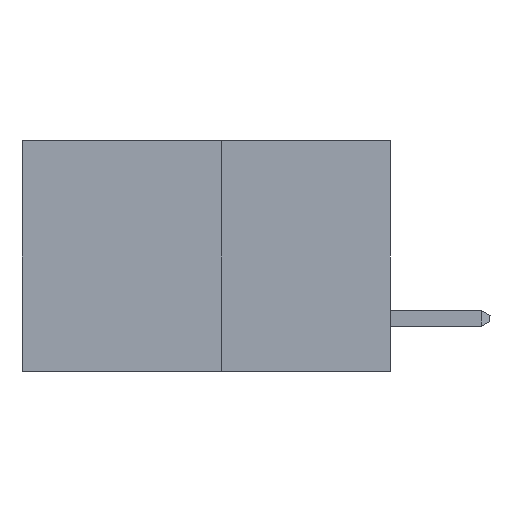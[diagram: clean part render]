
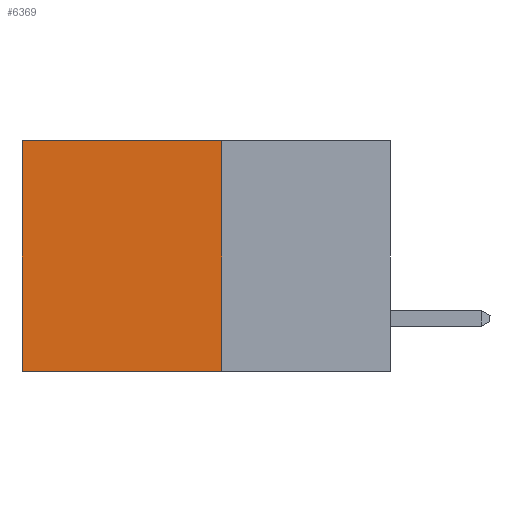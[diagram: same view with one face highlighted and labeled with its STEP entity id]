
A CAD part, left-side view. The second image highlights one B-rep face of the part: STEP entity #6369.
In plain terms, the highlighted planar face has unit normal (-1, 0, 0).
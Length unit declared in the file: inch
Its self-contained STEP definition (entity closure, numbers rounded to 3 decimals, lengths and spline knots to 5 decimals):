
#111 = LINE ( 'NONE', #5739, #2231 ) ;
#535 = VECTOR ( 'NONE', #11121, 39.37008 ) ;
#651 = CARTESIAN_POINT ( 'NONE',  ( 0.277, 0.59, -0.37 ) ) ;
#1813 = VERTEX_POINT ( 'NONE', #6706 ) ;
#1990 = DIRECTION ( 'NONE',  ( 0., 0., -1. ) ) ;
#1997 = DIRECTION ( 'NONE',  ( 1., 0., 0. ) ) ;
#2011 = CARTESIAN_POINT ( 'NONE',  ( 0.277, 0.27, -0.37 ) ) ;
#2077 = PLANE ( 'NONE',  #5406 ) ;
#2231 = VECTOR ( 'NONE', #9826, 39.37008 ) ;
#2453 = VERTEX_POINT ( 'NONE', #6259 ) ;
#2964 = LINE ( 'NONE', #9458, #535 ) ;
#3350 = VERTEX_POINT ( 'NONE', #651 ) ;
#3394 = LINE ( 'NONE', #5574, #9706 ) ;
#3421 = VERTEX_POINT ( 'NONE', #5643 ) ;
#5173 = LINE ( 'NONE', #9496, #9310 ) ;
#5353 = EDGE_LOOP ( 'NONE', ( #5484, #9858, #5751, #7945 ) ) ;
#5397 = DIRECTION ( 'NONE',  ( 0., 1., 0. ) ) ;
#5406 = AXIS2_PLACEMENT_3D ( 'NONE', #2011, #1997, #1990 ) ;
#5484 = ORIENTED_EDGE ( 'NONE', *, *, #7040, .T. ) ;
#5492 = FACE_OUTER_BOUND ( 'NONE', #5353, .T. ) ;
#5574 = CARTESIAN_POINT ( 'NONE',  ( 0.277, 0.27, -0.37 ) ) ;
#5643 = CARTESIAN_POINT ( 'NONE',  ( 0.277, 0.59, 0. ) ) ;
#5739 = CARTESIAN_POINT ( 'NONE',  ( 0.277, 0.59, -0.37 ) ) ;
#5751 = ORIENTED_EDGE ( 'NONE', *, *, #8072, .F. ) ;
#6259 = CARTESIAN_POINT ( 'NONE',  ( 0.277, 0.27, 0. ) ) ;
#6369 = ADVANCED_FACE ( 'NONE', ( #5492 ), #2077, .F. ) ;
#6396 = DIRECTION ( 'NONE',  ( 0., 0., -1. ) ) ;
#6706 = CARTESIAN_POINT ( 'NONE',  ( 0.277, 0.27, -0.37 ) ) ;
#7040 = EDGE_CURVE ( 'NONE', #3421, #3350, #111, .T. ) ;
#7945 = ORIENTED_EDGE ( 'NONE', *, *, #11094, .T. ) ;
#8072 = EDGE_CURVE ( 'NONE', #2453, #1813, #3394, .T. ) ;
#9310 = VECTOR ( 'NONE', #5397, 39.37008 ) ;
#9458 = CARTESIAN_POINT ( 'NONE',  ( 0.277, 0.27, -0.37 ) ) ;
#9496 = CARTESIAN_POINT ( 'NONE',  ( 0.277, 0.27, 0. ) ) ;
#9706 = VECTOR ( 'NONE', #6396, 39.37008 ) ;
#9826 = DIRECTION ( 'NONE',  ( 0., 0., -1. ) ) ;
#9858 = ORIENTED_EDGE ( 'NONE', *, *, #11073, .F. ) ;
#11073 = EDGE_CURVE ( 'NONE', #1813, #3350, #2964, .T. ) ;
#11094 = EDGE_CURVE ( 'NONE', #2453, #3421, #5173, .T. ) ;
#11121 = DIRECTION ( 'NONE',  ( 0., 1., 0. ) ) ;
